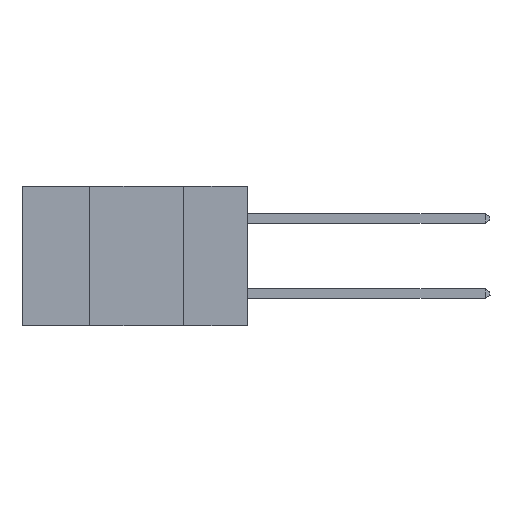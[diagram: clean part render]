
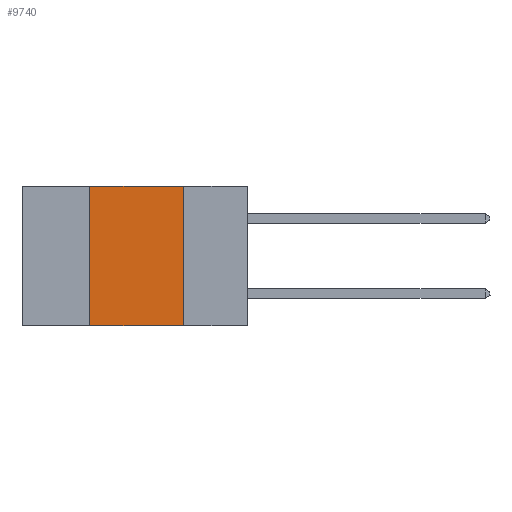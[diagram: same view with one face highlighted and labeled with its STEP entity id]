
A CAD part, left-side view. The second image highlights one B-rep face of the part: STEP entity #9740.
In plain terms, the highlighted planar face has unit normal (-1, 0, 0).
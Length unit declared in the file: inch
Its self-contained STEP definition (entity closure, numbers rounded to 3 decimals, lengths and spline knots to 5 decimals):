
#320 = PLANE ( 'NONE',  #9958 ) ;
#544 = DIRECTION ( 'NONE',  ( 1., 0., 0. ) ) ;
#803 = VERTEX_POINT ( 'NONE', #22097 ) ;
#805 = EDGE_CURVE ( 'NONE', #10852, #20593, #10983, .T. ) ;
#906 = CARTESIAN_POINT ( 'NONE',  ( 0., 0.42, 0. ) ) ;
#1502 = LINE ( 'NONE', #906, #5692 ) ;
#2274 = DIRECTION ( 'NONE',  ( 0., 0., -1. ) ) ;
#4092 = EDGE_LOOP ( 'NONE', ( #6646, #8507, #5682, #18892 ) ) ;
#4179 = VECTOR ( 'NONE', #18799, 39.37008 ) ;
#5498 = VERTEX_POINT ( 'NONE', #20921 ) ;
#5682 = ORIENTED_EDGE ( 'NONE', *, *, #13236, .F. ) ;
#5692 = VECTOR ( 'NONE', #15721, 39.37008 ) ;
#6646 = ORIENTED_EDGE ( 'NONE', *, *, #15654, .F. ) ;
#8507 = ORIENTED_EDGE ( 'NONE', *, *, #805, .F. ) ;
#9706 = DIRECTION ( 'NONE',  ( 0., -1., 0. ) ) ;
#9740 = ADVANCED_FACE ( 'NONE', ( #20241 ), #320, .F. ) ;
#9958 = AXIS2_PLACEMENT_3D ( 'NONE', #18155, #544, #2274 ) ;
#10852 = VERTEX_POINT ( 'NONE', #16407 ) ;
#10983 = LINE ( 'NONE', #20247, #12387 ) ;
#11558 = CARTESIAN_POINT ( 'NONE',  ( 0., 0.17, 0. ) ) ;
#11759 = EDGE_CURVE ( 'NONE', #5498, #803, #16905, .T. ) ;
#12387 = VECTOR ( 'NONE', #9706, 39.37008 ) ;
#12706 = DIRECTION ( 'NONE',  ( 0., -1., 0. ) ) ;
#13236 = EDGE_CURVE ( 'NONE', #5498, #10852, #1502, .T. ) ;
#15654 = EDGE_CURVE ( 'NONE', #20593, #803, #18374, .T. ) ;
#15721 = DIRECTION ( 'NONE',  ( 0., 0., 1. ) ) ;
#16248 = CARTESIAN_POINT ( 'NONE',  ( 0., 0.6, -0.37 ) ) ;
#16407 = CARTESIAN_POINT ( 'NONE',  ( 0., 0.42, 0. ) ) ;
#16905 = LINE ( 'NONE', #16248, #20767 ) ;
#18155 = CARTESIAN_POINT ( 'NONE',  ( 0., 0.6, 0. ) ) ;
#18374 = LINE ( 'NONE', #11558, #4179 ) ;
#18799 = DIRECTION ( 'NONE',  ( 0., 0., -1. ) ) ;
#18892 = ORIENTED_EDGE ( 'NONE', *, *, #11759, .T. ) ;
#19699 = CARTESIAN_POINT ( 'NONE',  ( 0., 0.17, 0. ) ) ;
#20241 = FACE_OUTER_BOUND ( 'NONE', #4092, .T. ) ;
#20247 = CARTESIAN_POINT ( 'NONE',  ( 0., 0.6, 0. ) ) ;
#20593 = VERTEX_POINT ( 'NONE', #19699 ) ;
#20767 = VECTOR ( 'NONE', #12706, 39.37008 ) ;
#20921 = CARTESIAN_POINT ( 'NONE',  ( 0., 0.42, -0.37 ) ) ;
#22097 = CARTESIAN_POINT ( 'NONE',  ( 0., 0.17, -0.37 ) ) ;
